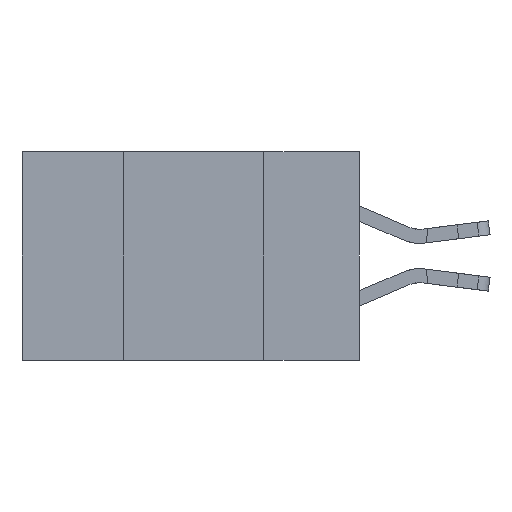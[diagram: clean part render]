
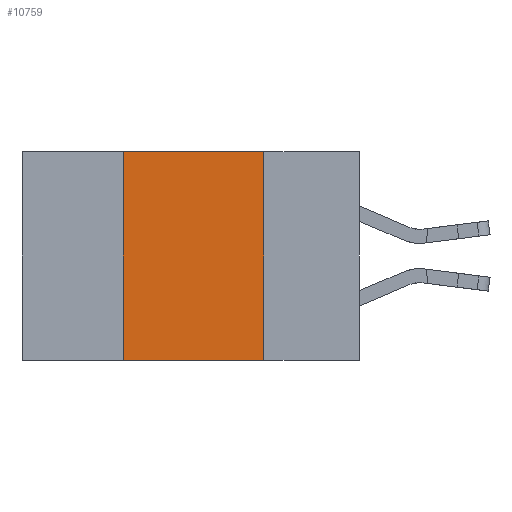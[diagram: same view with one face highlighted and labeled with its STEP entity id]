
A CAD part, left-side view. The second image highlights one B-rep face of the part: STEP entity #10759.
In plain terms, the highlighted planar face has unit normal (-1, 0, 0).
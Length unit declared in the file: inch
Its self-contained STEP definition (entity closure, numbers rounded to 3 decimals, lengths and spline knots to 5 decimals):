
#500 = CARTESIAN_POINT ( 'NONE',  ( 0., 0.42, 0. ) ) ;
#622 = DIRECTION ( 'NONE',  ( 0., -1., 0. ) ) ;
#932 = DIRECTION ( 'NONE',  ( 0., -1., 0. ) ) ;
#958 = CARTESIAN_POINT ( 'NONE',  ( 0., 0.17, 0. ) ) ;
#1101 = EDGE_CURVE ( 'NONE', #8570, #17263, #3211, .T. ) ;
#3033 = PLANE ( 'NONE',  #4235 ) ;
#3211 = LINE ( 'NONE', #8748, #12809 ) ;
#3259 = ORIENTED_EDGE ( 'NONE', *, *, #12526, .F. ) ;
#3832 = DIRECTION ( 'NONE',  ( 0., 0., -1. ) ) ;
#3973 = EDGE_CURVE ( 'NONE', #11492, #6307, #16413, .T. ) ;
#4235 = AXIS2_PLACEMENT_3D ( 'NONE', #16011, #10566, #3832 ) ;
#4527 = ORIENTED_EDGE ( 'NONE', *, *, #3973, .F. ) ;
#5157 = CARTESIAN_POINT ( 'NONE',  ( 0., 0.42, -0.37 ) ) ;
#5737 = ORIENTED_EDGE ( 'NONE', *, *, #8861, .F. ) ;
#5970 = DIRECTION ( 'NONE',  ( 0., 0., 1. ) ) ;
#6307 = VERTEX_POINT ( 'NONE', #958 ) ;
#7848 = EDGE_LOOP ( 'NONE', ( #3259, #4527, #5737, #16945 ) ) ;
#8570 = VERTEX_POINT ( 'NONE', #5157 ) ;
#8601 = LINE ( 'NONE', #500, #8818 ) ;
#8748 = CARTESIAN_POINT ( 'NONE',  ( 0., 0.6, -0.37 ) ) ;
#8818 = VECTOR ( 'NONE', #5970, 39.37008 ) ;
#8861 = EDGE_CURVE ( 'NONE', #8570, #11492, #8601, .T. ) ;
#9783 = VECTOR ( 'NONE', #932, 39.37008 ) ;
#10441 = CARTESIAN_POINT ( 'NONE',  ( 0., 0.6, 0. ) ) ;
#10566 = DIRECTION ( 'NONE',  ( 1., 0., 0. ) ) ;
#10759 = ADVANCED_FACE ( 'NONE', ( #16638 ), #3033, .F. ) ;
#11450 = LINE ( 'NONE', #12075, #12501 ) ;
#11492 = VERTEX_POINT ( 'NONE', #12747 ) ;
#12075 = CARTESIAN_POINT ( 'NONE',  ( 0., 0.17, 0. ) ) ;
#12501 = VECTOR ( 'NONE', #16332, 39.37008 ) ;
#12526 = EDGE_CURVE ( 'NONE', #6307, #17263, #11450, .T. ) ;
#12747 = CARTESIAN_POINT ( 'NONE',  ( 0., 0.42, 0. ) ) ;
#12809 = VECTOR ( 'NONE', #622, 39.37008 ) ;
#13851 = CARTESIAN_POINT ( 'NONE',  ( 0., 0.17, -0.37 ) ) ;
#16011 = CARTESIAN_POINT ( 'NONE',  ( 0., 0.6, 0. ) ) ;
#16332 = DIRECTION ( 'NONE',  ( 0., 0., -1. ) ) ;
#16413 = LINE ( 'NONE', #10441, #9783 ) ;
#16638 = FACE_OUTER_BOUND ( 'NONE', #7848, .T. ) ;
#16945 = ORIENTED_EDGE ( 'NONE', *, *, #1101, .T. ) ;
#17263 = VERTEX_POINT ( 'NONE', #13851 ) ;
